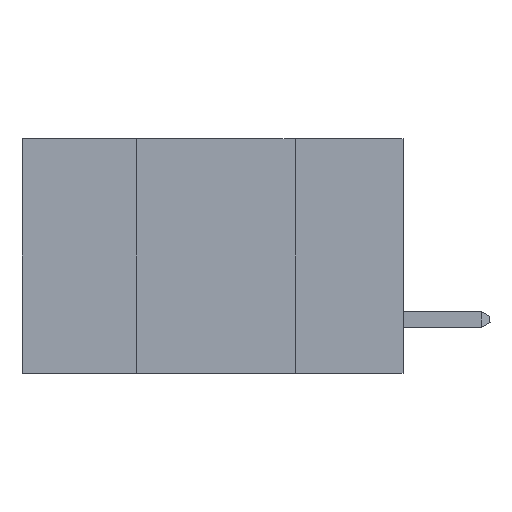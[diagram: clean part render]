
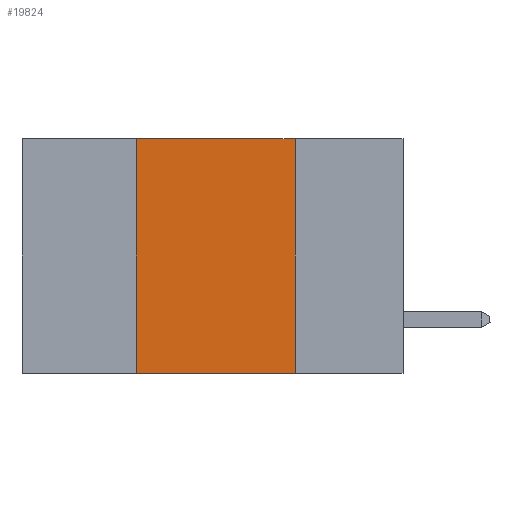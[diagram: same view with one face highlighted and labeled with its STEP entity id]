
A CAD part, left-side view. The second image highlights one B-rep face of the part: STEP entity #19824.
In plain terms, the highlighted planar face has unit normal (-1, 0, 0).
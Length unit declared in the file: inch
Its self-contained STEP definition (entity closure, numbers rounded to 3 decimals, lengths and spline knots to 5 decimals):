
#195 = CARTESIAN_POINT ( 'NONE',  ( 0., 0.6, 0. ) ) ;
#472 = EDGE_CURVE ( 'NONE', #17923, #11097, #17763, .T. ) ;
#3146 = EDGE_CURVE ( 'NONE', #11097, #18846, #8058, .T. ) ;
#3155 = FACE_OUTER_BOUND ( 'NONE', #12229, .T. ) ;
#3930 = LINE ( 'NONE', #19751, #23350 ) ;
#4573 = ORIENTED_EDGE ( 'NONE', *, *, #472, .F. ) ;
#6128 = CARTESIAN_POINT ( 'NONE',  ( 0., 0.42, -0.37 ) ) ;
#6280 = CARTESIAN_POINT ( 'NONE',  ( 0., 0.42, 0. ) ) ;
#6640 = CARTESIAN_POINT ( 'NONE',  ( 0., 0.6, 0. ) ) ;
#7172 = DIRECTION ( 'NONE',  ( 0., 0., -1. ) ) ;
#7176 = EDGE_CURVE ( 'NONE', #25366, #17923, #14977, .T. ) ;
#8058 = LINE ( 'NONE', #16048, #18994 ) ;
#9556 = EDGE_CURVE ( 'NONE', #25366, #18846, #3930, .T. ) ;
#10237 = DIRECTION ( 'NONE',  ( 0., -1., 0. ) ) ;
#11097 = VERTEX_POINT ( 'NONE', #14516 ) ;
#11170 = ORIENTED_EDGE ( 'NONE', *, *, #3146, .F. ) ;
#11382 = PLANE ( 'NONE',  #20701 ) ;
#12229 = EDGE_LOOP ( 'NONE', ( #11170, #4573, #23065, #22417 ) ) ;
#12716 = CARTESIAN_POINT ( 'NONE',  ( 0., 0.42, 0. ) ) ;
#13288 = DIRECTION ( 'NONE',  ( 1., 0., 0. ) ) ;
#14516 = CARTESIAN_POINT ( 'NONE',  ( 0., 0.17, 0. ) ) ;
#14977 = LINE ( 'NONE', #12716, #15703 ) ;
#15703 = VECTOR ( 'NONE', #22002, 39.37008 ) ;
#16048 = CARTESIAN_POINT ( 'NONE',  ( 0., 0.17, 0. ) ) ;
#17763 = LINE ( 'NONE', #195, #18417 ) ;
#17923 = VERTEX_POINT ( 'NONE', #6280 ) ;
#18417 = VECTOR ( 'NONE', #10237, 39.37008 ) ;
#18846 = VERTEX_POINT ( 'NONE', #22246 ) ;
#18994 = VECTOR ( 'NONE', #7172, 39.37008 ) ;
#19751 = CARTESIAN_POINT ( 'NONE',  ( 0., 0.6, -0.37 ) ) ;
#19824 = ADVANCED_FACE ( 'NONE', ( #3155 ), #11382, .F. ) ;
#20701 = AXIS2_PLACEMENT_3D ( 'NONE', #6640, #13288, #27070 ) ;
#22002 = DIRECTION ( 'NONE',  ( 0., 0., 1. ) ) ;
#22246 = CARTESIAN_POINT ( 'NONE',  ( 0., 0.17, -0.37 ) ) ;
#22417 = ORIENTED_EDGE ( 'NONE', *, *, #9556, .T. ) ;
#23065 = ORIENTED_EDGE ( 'NONE', *, *, #7176, .F. ) ;
#23350 = VECTOR ( 'NONE', #28854, 39.37008 ) ;
#25366 = VERTEX_POINT ( 'NONE', #6128 ) ;
#27070 = DIRECTION ( 'NONE',  ( 0., 0., -1. ) ) ;
#28854 = DIRECTION ( 'NONE',  ( 0., -1., 0. ) ) ;
